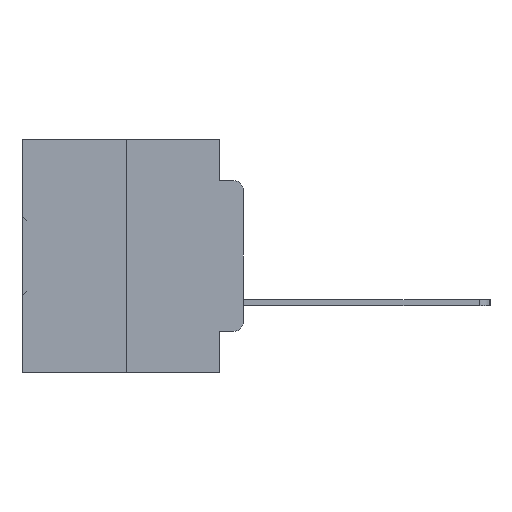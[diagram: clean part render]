
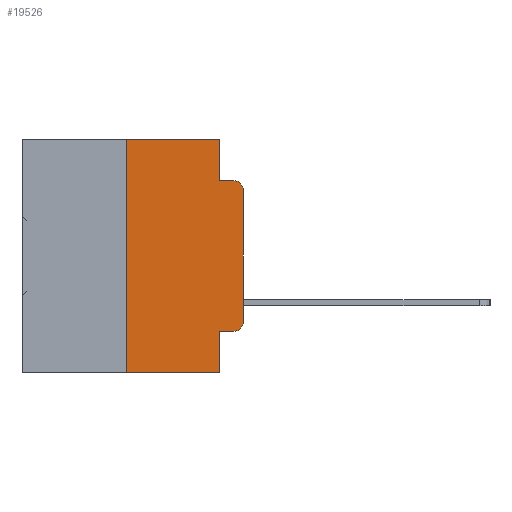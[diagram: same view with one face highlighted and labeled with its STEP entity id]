
A CAD part, left-side view. The second image highlights one B-rep face of the part: STEP entity #19526.
In plain terms, the highlighted planar face has unit normal (-1, 0, 0).
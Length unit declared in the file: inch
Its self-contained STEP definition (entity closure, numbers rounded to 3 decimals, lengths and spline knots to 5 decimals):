
#286 = VECTOR ( 'NONE', #5888, 39.37008 ) ;
#555 = CARTESIAN_POINT ( 'NONE',  ( 0., 0.051, -0.0885 ) ) ;
#557 = DIRECTION ( 'NONE',  ( 0., 0., -1. ) ) ;
#1569 = EDGE_CURVE ( 'NONE', #4714, #17348, #9388, .T. ) ;
#1598 = VERTEX_POINT ( 'NONE', #7388 ) ;
#2068 = CARTESIAN_POINT ( 'NONE',  ( 0., 0.25, 0. ) ) ;
#2642 = VECTOR ( 'NONE', #4593, 39.37008 ) ;
#2846 = VECTOR ( 'NONE', #23504, 39.37008 ) ;
#3093 = VERTEX_POINT ( 'NONE', #2068 ) ;
#3417 = EDGE_CURVE ( 'NONE', #17348, #11585, #8859, .T. ) ;
#3674 = EDGE_CURVE ( 'NONE', #3093, #4714, #15666, .T. ) ;
#4219 = CARTESIAN_POINT ( 'NONE',  ( 0., 0.473, -0.5 ) ) ;
#4593 = DIRECTION ( 'NONE',  ( 0., 0., -1. ) ) ;
#4625 = ORIENTED_EDGE ( 'NONE', *, *, #10849, .T. ) ;
#4714 = VERTEX_POINT ( 'NONE', #14811 ) ;
#4879 = ORIENTED_EDGE ( 'NONE', *, *, #5268, .T. ) ;
#5200 = CARTESIAN_POINT ( 'NONE',  ( 0., 0.02, -0.3915 ) ) ;
#5268 = EDGE_CURVE ( 'NONE', #10037, #11585, #26013, .T. ) ;
#5315 = ORIENTED_EDGE ( 'NONE', *, *, #3417, .F. ) ;
#5367 = ORIENTED_EDGE ( 'NONE', *, *, #1569, .F. ) ;
#5637 = ORIENTED_EDGE ( 'NONE', *, *, #3674, .F. ) ;
#5673 = ORIENTED_EDGE ( 'NONE', *, *, #27724, .F. ) ;
#5827 = DIRECTION ( 'NONE',  ( 0., -1., 0. ) ) ;
#5889 = ORIENTED_EDGE ( 'NONE', *, *, #7652, .T. ) ;
#5888 = DIRECTION ( 'NONE',  ( 0., 0., 1. ) ) ;
#6166 = AXIS2_PLACEMENT_3D ( 'NONE', #5200, #24229, #8027 ) ;
#6173 = CARTESIAN_POINT ( 'NONE',  ( 0., 0.02, -0.4115 ) ) ;
#6366 = VERTEX_POINT ( 'NONE', #9423 ) ;
#6667 = LINE ( 'NONE', #29237, #34374 ) ;
#7135 = ORIENTED_EDGE ( 'NONE', *, *, #24184, .F. ) ;
#7388 = CARTESIAN_POINT ( 'NONE',  ( 0., 0.25, -0.5 ) ) ;
#7508 = ORIENTED_EDGE ( 'NONE', *, *, #22381, .T. ) ;
#7598 = ORIENTED_EDGE ( 'NONE', *, *, #16983, .T. ) ;
#7652 = EDGE_CURVE ( 'NONE', #1598, #21313, #24189, .T. ) ;
#7920 = CARTESIAN_POINT ( 'NONE',  ( 0., 0.051, -0.4115 ) ) ;
#8027 = DIRECTION ( 'NONE',  ( 0., 0., -1. ) ) ;
#8859 = LINE ( 'NONE', #22007, #29477 ) ;
#9009 = DIRECTION ( 'NONE',  ( 0., -1., 0. ) ) ;
#9388 = LINE ( 'NONE', #20812, #2846 ) ;
#9423 = CARTESIAN_POINT ( 'NONE',  ( 0., 0., -0.3915 ) ) ;
#10037 = VERTEX_POINT ( 'NONE', #28979 ) ;
#10295 = VERTEX_POINT ( 'NONE', #6173 ) ;
#10454 = CARTESIAN_POINT ( 'NONE',  ( 0., 0.051, -0.4115 ) ) ;
#10849 = EDGE_CURVE ( 'NONE', #6366, #10037, #22998, .T. ) ;
#10975 = AXIS2_PLACEMENT_3D ( 'NONE', #20118, #12078, #557 ) ;
#11585 = VERTEX_POINT ( 'NONE', #29888 ) ;
#11733 = LINE ( 'NONE', #18266, #2642 ) ;
#12078 = DIRECTION ( 'NONE',  ( -1., 0., 0. ) ) ;
#13170 = DIRECTION ( 'NONE',  ( 0., 0., 1. ) ) ;
#13588 = DIRECTION ( 'NONE',  ( 1., 0., 0. ) ) ;
#14811 = CARTESIAN_POINT ( 'NONE',  ( 0., 0.051, 0. ) ) ;
#15666 = LINE ( 'NONE', #33359, #28223 ) ;
#16677 = CARTESIAN_POINT ( 'NONE',  ( 0., 0.051, -0.5 ) ) ;
#16983 = EDGE_CURVE ( 'NONE', #10295, #6366, #20482, .T. ) ;
#17043 = VECTOR ( 'NONE', #25966, 39.37008 ) ;
#17348 = VERTEX_POINT ( 'NONE', #555 ) ;
#17886 = EDGE_LOOP ( 'NONE', ( #4625, #4879, #5315, #5367, #5637, #5673, #5889, #7135, #7508, #7598 ) ) ;
#18266 = CARTESIAN_POINT ( 'NONE',  ( 0., 0.051, 0. ) ) ;
#18924 = PLANE ( 'NONE',  #31483 ) ;
#19526 = ADVANCED_FACE ( 'NONE', ( #21939 ), #18924, .F. ) ;
#20118 = CARTESIAN_POINT ( 'NONE',  ( 0., 0.02, -0.1085 ) ) ;
#20482 = CIRCLE ( 'NONE', #6166, 0.02 ) ;
#20812 = CARTESIAN_POINT ( 'NONE',  ( 0., 0.051, 0. ) ) ;
#21313 = VERTEX_POINT ( 'NONE', #16677 ) ;
#21785 = VECTOR ( 'NONE', #32079, 39.37008 ) ;
#21939 = FACE_OUTER_BOUND ( 'NONE', #17886, .T. ) ;
#22007 = CARTESIAN_POINT ( 'NONE',  ( 0., 0.051, -0.0885 ) ) ;
#22381 = EDGE_CURVE ( 'NONE', #25881, #10295, #22644, .T. ) ;
#22644 = LINE ( 'NONE', #7920, #21785 ) ;
#22998 = LINE ( 'NONE', #30064, #286 ) ;
#23504 = DIRECTION ( 'NONE',  ( 0., 0., -1. ) ) ;
#24184 = EDGE_CURVE ( 'NONE', #25881, #21313, #11733, .T. ) ;
#24189 = LINE ( 'NONE', #4219, #17043 ) ;
#24229 = DIRECTION ( 'NONE',  ( -1., 0., 0. ) ) ;
#25881 = VERTEX_POINT ( 'NONE', #10454 ) ;
#25966 = DIRECTION ( 'NONE',  ( 0., -1., 0. ) ) ;
#26013 = CIRCLE ( 'NONE', #10975, 0.02 ) ;
#26986 = CARTESIAN_POINT ( 'NONE',  ( 0., 0.473, 0. ) ) ;
#27724 = EDGE_CURVE ( 'NONE', #1598, #3093, #6667, .T. ) ;
#28223 = VECTOR ( 'NONE', #5827, 39.37008 ) ;
#28979 = CARTESIAN_POINT ( 'NONE',  ( 0., 0., -0.1085 ) ) ;
#29237 = CARTESIAN_POINT ( 'NONE',  ( 0., 0.25, 0. ) ) ;
#29477 = VECTOR ( 'NONE', #9009, 39.37008 ) ;
#29888 = CARTESIAN_POINT ( 'NONE',  ( 0., 0.02, -0.0885 ) ) ;
#30064 = CARTESIAN_POINT ( 'NONE',  ( 0., 0., 0. ) ) ;
#31483 = AXIS2_PLACEMENT_3D ( 'NONE', #26986, #13588, #32250 ) ;
#32079 = DIRECTION ( 'NONE',  ( 0., -1., 0. ) ) ;
#32250 = DIRECTION ( 'NONE',  ( 0., 0., -1. ) ) ;
#33359 = CARTESIAN_POINT ( 'NONE',  ( 0., 0.473, 0. ) ) ;
#34374 = VECTOR ( 'NONE', #13170, 39.37008 ) ;
